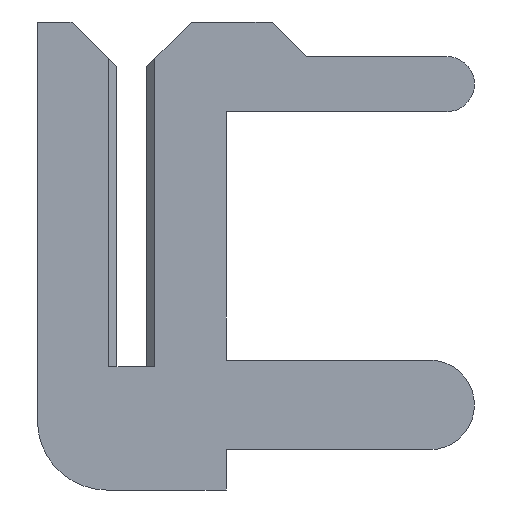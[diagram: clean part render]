
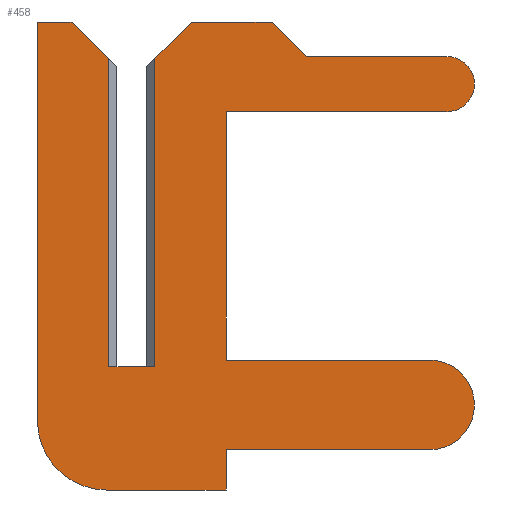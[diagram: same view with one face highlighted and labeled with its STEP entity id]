
A CAD part, left-side view. The second image highlights one B-rep face of the part: STEP entity #458.
In plain terms, the highlighted planar face has unit normal (-1, 0, 0).
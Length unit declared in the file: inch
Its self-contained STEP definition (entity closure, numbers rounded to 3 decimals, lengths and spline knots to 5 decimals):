
#7 = ORIENTED_EDGE ( 'NONE', *, *, #268, .F. ) ;
#10 = CARTESIAN_POINT ( 'NONE',  ( -0.01, -0.041, 0.003 ) ) ;
#18 = CARTESIAN_POINT ( 'NONE',  ( -0.01, -0.1295, 0.003 ) ) ;
#25 = VERTEX_POINT ( 'NONE', #634 ) ;
#36 = AXIS2_PLACEMENT_3D ( 'NONE', #259, #70, #266 ) ;
#47 = DIRECTION ( 'NONE',  ( 0., -0.707, -0.707 ) ) ;
#51 = EDGE_CURVE ( 'NONE', #281, #777, #985, .T. ) ;
#63 = ORIENTED_EDGE ( 'NONE', *, *, #945, .F. ) ;
#70 = DIRECTION ( 'NONE',  ( 1., 0., 0. ) ) ;
#98 = LINE ( 'NONE', #892, #1042 ) ;
#109 = DIRECTION ( 'NONE',  ( 0., 0., 1. ) ) ;
#126 = ORIENTED_EDGE ( 'NONE', *, *, #861, .F. ) ;
#150 = DIRECTION ( 'NONE',  ( 0., 0., 1. ) ) ;
#153 = ORIENTED_EDGE ( 'NONE', *, *, #195, .F. ) ;
#160 = EDGE_CURVE ( 'NONE', #1071, #261, #999, .T. ) ;
#163 = AXIS2_PLACEMENT_3D ( 'NONE', #726, #637, #150 ) ;
#188 = ORIENTED_EDGE ( 'NONE', *, *, #512, .T. ) ;
#193 = ORIENTED_EDGE ( 'NONE', *, *, #51, .F. ) ;
#195 = EDGE_CURVE ( 'NONE', #754, #1014, #1175, .T. ) ;
#213 = CARTESIAN_POINT ( 'NONE',  ( -0.01, -0.026, 0.15 ) ) ;
#217 = ORIENTED_EDGE ( 'NONE', *, *, #635, .F. ) ;
#218 = CIRCLE ( 'NONE', #833, 0.012 ) ;
#219 = AXIS2_PLACEMENT_3D ( 'NONE', #499, #789, #887 ) ;
#239 = EDGE_CURVE ( 'NONE', #1014, #1182, #761, .T. ) ;
#243 = ORIENTED_EDGE ( 'NONE', *, *, #272, .F. ) ;
#251 = VECTOR ( 'NONE', #1224, 39.37008 ) ;
#252 = LINE ( 'NONE', #551, #1010 ) ;
#259 = CARTESIAN_POINT ( 'NONE',  ( -0.01, -0.1295, -0.0165 ) ) ;
#260 = CARTESIAN_POINT ( 'NONE',  ( -0.01, -0.041, 0.003 ) ) ;
#261 = VERTEX_POINT ( 'NONE', #481 ) ;
#266 = DIRECTION ( 'NONE',  ( 0., 0., 1. ) ) ;
#267 = CARTESIAN_POINT ( 'NONE',  ( -0.01, -0.01, 0.15 ) ) ;
#268 = EDGE_CURVE ( 'NONE', #298, #1227, #570, .T. ) ;
#272 = EDGE_CURVE ( 'NONE', #704, #25, #252, .T. ) ;
#279 = VECTOR ( 'NONE', #881, 39.37008 ) ;
#281 = VERTEX_POINT ( 'NONE', #839 ) ;
#282 = DIRECTION ( 'NONE',  ( 0., 0., -1. ) ) ;
#298 = VERTEX_POINT ( 'NONE', #1053 ) ;
#304 = CARTESIAN_POINT ( 'NONE',  ( -0.01, 0.011, -0.0535 ) ) ;
#311 = DIRECTION ( 'NONE',  ( 0., -1., 0. ) ) ;
#374 = DIRECTION ( 'NONE',  ( 0., -1., 0. ) ) ;
#403 = CARTESIAN_POINT ( 'NONE',  ( -0.01, -0.137, 0.111 ) ) ;
#407 = PLANE ( 'NONE',  #219 ) ;
#408 = VECTOR ( 'NONE', #654, 39.37008 ) ;
#416 = ORIENTED_EDGE ( 'NONE', *, *, #806, .F. ) ;
#428 = ORIENTED_EDGE ( 'NONE', *, *, #1032, .F. ) ;
#433 = CARTESIAN_POINT ( 'NONE',  ( -0.01, -0.076, 0.135 ) ) ;
#439 = DIRECTION ( 'NONE',  ( 0., 0., 1. ) ) ;
#444 = EDGE_CURVE ( 'NONE', #777, #1048, #1062, .T. ) ;
#447 = CARTESIAN_POINT ( 'NONE',  ( -0.01, -0.137, 0.135 ) ) ;
#457 = ORIENTED_EDGE ( 'NONE', *, *, #1159, .F. ) ;
#458 = ADVANCED_FACE ( 'NONE', ( #858 ), #407, .T. ) ;
#467 = CARTESIAN_POINT ( 'NONE',  ( -0.01, -0.041, 0.111 ) ) ;
#481 = CARTESIAN_POINT ( 'NONE',  ( -0.01, -0.01, 0. ) ) ;
#482 = CARTESIAN_POINT ( 'NONE',  ( -0.01, -0.026, 0.15 ) ) ;
#499 = CARTESIAN_POINT ( 'NONE',  ( -0.01, 0.011, -0.0235 ) ) ;
#512 = EDGE_CURVE ( 'NONE', #1071, #995, #98, .T. ) ;
#514 = EDGE_CURVE ( 'NONE', #25, #771, #711, .T. ) ;
#527 = EDGE_CURVE ( 'NONE', #625, #995, #929, .T. ) ;
#538 = CARTESIAN_POINT ( 'NONE',  ( -0.01, -0.041, -0.036 ) ) ;
#551 = CARTESIAN_POINT ( 'NONE',  ( -0.01, -0.041, -0.0535 ) ) ;
#560 = VECTOR ( 'NONE', #439, 39.37008 ) ;
#570 = LINE ( 'NONE', #1232, #1056 ) ;
#577 = ORIENTED_EDGE ( 'NONE', *, *, #444, .F. ) ;
#581 = EDGE_CURVE ( 'NONE', #1008, #622, #1087, .T. ) ;
#594 = CARTESIAN_POINT ( 'NONE',  ( -0.01, 0.026, 0.15 ) ) ;
#622 = VERTEX_POINT ( 'NONE', #1210 ) ;
#625 = VERTEX_POINT ( 'NONE', #916 ) ;
#634 = CARTESIAN_POINT ( 'NONE',  ( -0.01, -0.041, -0.0535 ) ) ;
#635 = EDGE_CURVE ( 'NONE', #1048, #298, #651, .T. ) ;
#637 = DIRECTION ( 'NONE',  ( 1., 0., 0. ) ) ;
#646 = DIRECTION ( 'NONE',  ( 0., -1., 0. ) ) ;
#651 = LINE ( 'NONE', #433, #1135 ) ;
#654 = DIRECTION ( 'NONE',  ( 0., -1., 0. ) ) ;
#659 = DIRECTION ( 'NONE',  ( 0., 0., -1. ) ) ;
#674 = ORIENTED_EDGE ( 'NONE', *, *, #1134, .F. ) ;
#691 = VECTOR ( 'NONE', #1054, 39.37008 ) ;
#692 = ORIENTED_EDGE ( 'NONE', *, *, #581, .F. ) ;
#699 = VECTOR ( 'NONE', #1073, 39.37008 ) ;
#704 = VERTEX_POINT ( 'NONE', #538 ) ;
#708 = EDGE_CURVE ( 'NONE', #281, #261, #1117, .T. ) ;
#711 = LINE ( 'NONE', #304, #699 ) ;
#718 = VECTOR ( 'NONE', #993, 39.37008 ) ;
#724 = VECTOR ( 'NONE', #646, 39.37008 ) ;
#726 = CARTESIAN_POINT ( 'NONE',  ( -0.01, 0.011, -0.0235 ) ) ;
#728 = CARTESIAN_POINT ( 'NONE',  ( -0.01, 0.0065, 0.1305 ) ) ;
#729 = VECTOR ( 'NONE', #311, 39.37008 ) ;
#739 = CARTESIAN_POINT ( 'NONE',  ( -0.01, 0.041, 0.15 ) ) ;
#754 = VERTEX_POINT ( 'NONE', #941 ) ;
#761 = LINE ( 'NONE', #953, #724 ) ;
#762 = ORIENTED_EDGE ( 'NONE', *, *, #708, .T. ) ;
#771 = VERTEX_POINT ( 'NONE', #1147 ) ;
#777 = VERTEX_POINT ( 'NONE', #482 ) ;
#789 = DIRECTION ( 'NONE',  ( -1., 0., 0. ) ) ;
#801 = CIRCLE ( 'NONE', #163, 0.03 ) ;
#803 = ORIENTED_EDGE ( 'NONE', *, *, #527, .F. ) ;
#806 = EDGE_CURVE ( 'NONE', #909, #754, #877, .T. ) ;
#825 = LINE ( 'NONE', #594, #279 ) ;
#833 = AXIS2_PLACEMENT_3D ( 'NONE', #1161, #984, #109 ) ;
#839 = CARTESIAN_POINT ( 'NONE',  ( -0.01, -0.01, 0.134 ) ) ;
#855 = CARTESIAN_POINT ( 'NONE',  ( -0.01, 0.0065, 0. ) ) ;
#858 = FACE_OUTER_BOUND ( 'NONE', #1093, .T. ) ;
#861 = EDGE_CURVE ( 'NONE', #1227, #909, #218, .T. ) ;
#864 = VECTOR ( 'NONE', #1238, 39.37008 ) ;
#870 = DIRECTION ( 'NONE',  ( 0., 0., 1. ) ) ;
#877 = LINE ( 'NONE', #467, #691 ) ;
#881 = DIRECTION ( 'NONE',  ( 0., -1., 0. ) ) ;
#887 = DIRECTION ( 'NONE',  ( 0., 0., 1. ) ) ;
#892 = CARTESIAN_POINT ( 'NONE',  ( -0.01, 0.01, -0.0235 ) ) ;
#909 = VERTEX_POINT ( 'NONE', #403 ) ;
#915 = VECTOR ( 'NONE', #282, 39.37008 ) ;
#916 = CARTESIAN_POINT ( 'NONE',  ( -0.01, 0.026, 0.15 ) ) ;
#929 = LINE ( 'NONE', #728, #251 ) ;
#933 = CARTESIAN_POINT ( 'NONE',  ( -0.01, -0.1295, -0.036 ) ) ;
#941 = CARTESIAN_POINT ( 'NONE',  ( -0.01, -0.041, 0.111 ) ) ;
#945 = EDGE_CURVE ( 'NONE', #622, #625, #825, .T. ) ;
#953 = CARTESIAN_POINT ( 'NONE',  ( -0.01, -0.1295, 0.003 ) ) ;
#984 = DIRECTION ( 'NONE',  ( 1., 0., 0. ) ) ;
#985 = LINE ( 'NONE', #1036, #1250 ) ;
#993 = DIRECTION ( 'NONE',  ( 0., 1., 0. ) ) ;
#995 = VERTEX_POINT ( 'NONE', #1086 ) ;
#999 = LINE ( 'NONE', #855, #408 ) ;
#1008 = VERTEX_POINT ( 'NONE', #1201 ) ;
#1010 = VECTOR ( 'NONE', #659, 39.37008 ) ;
#1014 = VERTEX_POINT ( 'NONE', #10 ) ;
#1015 = CIRCLE ( 'NONE', #36, 0.0195 ) ;
#1032 = EDGE_CURVE ( 'NONE', #1170, #704, #1094, .T. ) ;
#1036 = CARTESIAN_POINT ( 'NONE',  ( -0.01, -0.0065, 0.1305 ) ) ;
#1042 = VECTOR ( 'NONE', #870, 39.37008 ) ;
#1048 = VERTEX_POINT ( 'NONE', #1095 ) ;
#1053 = CARTESIAN_POINT ( 'NONE',  ( -0.01, -0.076, 0.135 ) ) ;
#1054 = DIRECTION ( 'NONE',  ( 0., 1., 0. ) ) ;
#1056 = VECTOR ( 'NONE', #374, 39.37008 ) ;
#1062 = LINE ( 'NONE', #213, #729 ) ;
#1071 = VERTEX_POINT ( 'NONE', #1082 ) ;
#1073 = DIRECTION ( 'NONE',  ( 0., 1., 0. ) ) ;
#1082 = CARTESIAN_POINT ( 'NONE',  ( -0.01, 0.01, 0. ) ) ;
#1086 = CARTESIAN_POINT ( 'NONE',  ( -0.01, 0.01, 0.134 ) ) ;
#1087 = LINE ( 'NONE', #739, #560 ) ;
#1093 = EDGE_LOOP ( 'NONE', ( #193, #762, #1115, #188, #803, #63, #692, #674, #1144, #243, #428, #457, #1166, #153, #416, #126, #7, #217, #577 ) ) ;
#1094 = LINE ( 'NONE', #1177, #718 ) ;
#1095 = CARTESIAN_POINT ( 'NONE',  ( -0.01, -0.061, 0.15 ) ) ;
#1115 = ORIENTED_EDGE ( 'NONE', *, *, #160, .F. ) ;
#1117 = LINE ( 'NONE', #267, #864 ) ;
#1134 = EDGE_CURVE ( 'NONE', #771, #1008, #801, .T. ) ;
#1135 = VECTOR ( 'NONE', #47, 39.37008 ) ;
#1144 = ORIENTED_EDGE ( 'NONE', *, *, #514, .F. ) ;
#1147 = CARTESIAN_POINT ( 'NONE',  ( -0.01, 0.011, -0.0535 ) ) ;
#1159 = EDGE_CURVE ( 'NONE', #1182, #1170, #1015, .T. ) ;
#1161 = CARTESIAN_POINT ( 'NONE',  ( -0.01, -0.137, 0.123 ) ) ;
#1166 = ORIENTED_EDGE ( 'NONE', *, *, #239, .F. ) ;
#1170 = VERTEX_POINT ( 'NONE', #933 ) ;
#1175 = LINE ( 'NONE', #260, #915 ) ;
#1177 = CARTESIAN_POINT ( 'NONE',  ( -0.01, -0.041, -0.036 ) ) ;
#1182 = VERTEX_POINT ( 'NONE', #18 ) ;
#1201 = CARTESIAN_POINT ( 'NONE',  ( -0.01, 0.041, -0.0235 ) ) ;
#1210 = CARTESIAN_POINT ( 'NONE',  ( -0.01, 0.041, 0.15 ) ) ;
#1212 = DIRECTION ( 'NONE',  ( 0., -0.707, 0.707 ) ) ;
#1224 = DIRECTION ( 'NONE',  ( 0., -0.707, -0.707 ) ) ;
#1227 = VERTEX_POINT ( 'NONE', #447 ) ;
#1232 = CARTESIAN_POINT ( 'NONE',  ( -0.01, -0.137, 0.135 ) ) ;
#1238 = DIRECTION ( 'NONE',  ( 0., 0., -1. ) ) ;
#1250 = VECTOR ( 'NONE', #1212, 39.37008 ) ;
